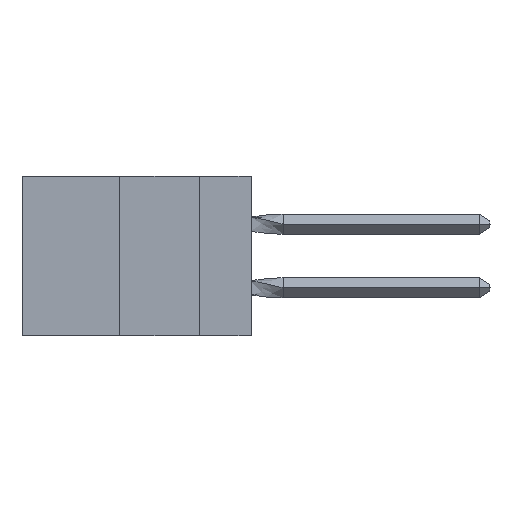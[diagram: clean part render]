
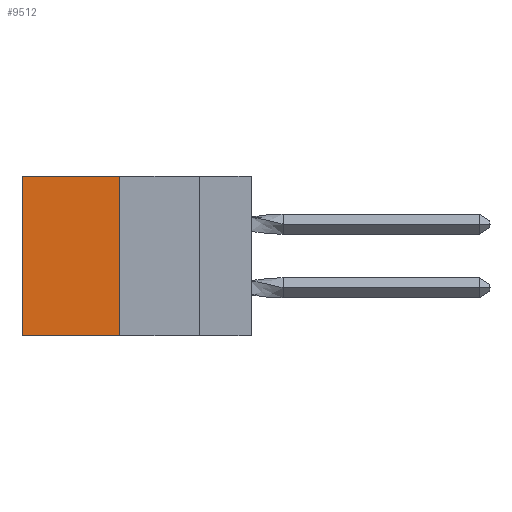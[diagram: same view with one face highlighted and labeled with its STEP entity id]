
A CAD part, left-side view. The second image highlights one B-rep face of the part: STEP entity #9512.
In plain terms, the highlighted planar face has unit normal (-1, 0, 0).
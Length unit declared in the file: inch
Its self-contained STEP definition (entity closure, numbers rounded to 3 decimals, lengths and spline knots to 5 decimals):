
#58 = VERTEX_POINT ( 'NONE', #33733 ) ;
#364 = CARTESIAN_POINT ( 'NONE',  ( 0.305, 0.413, 0. ) ) ;
#614 = PLANE ( 'NONE',  #31232 ) ;
#2203 = EDGE_CURVE ( 'NONE', #58, #4278, #3435, .T. ) ;
#2851 = DIRECTION ( 'NONE',  ( 1., 0., 0. ) ) ;
#3077 = DIRECTION ( 'NONE',  ( 0., 0., -1. ) ) ;
#3435 = LINE ( 'NONE', #13262, #12978 ) ;
#4278 = VERTEX_POINT ( 'NONE', #6064 ) ;
#4628 = CARTESIAN_POINT ( 'NONE',  ( 0.305, 0.72, -0.5 ) ) ;
#5631 = EDGE_CURVE ( 'NONE', #26437, #21655, #18759, .T. ) ;
#6064 = CARTESIAN_POINT ( 'NONE',  ( 0.305, 0.413, -0.5 ) ) ;
#6099 = FACE_OUTER_BOUND ( 'NONE', #22863, .T. ) ;
#6787 = CARTESIAN_POINT ( 'NONE',  ( 0.305, 0.72, 0. ) ) ;
#9512 = ADVANCED_FACE ( 'NONE', ( #6099 ), #614, .F. ) ;
#11023 = CARTESIAN_POINT ( 'NONE',  ( 0.305, 0.413, -0.5 ) ) ;
#11597 = VECTOR ( 'NONE', #33432, 39.37008 ) ;
#12978 = VECTOR ( 'NONE', #21033, 39.37008 ) ;
#13262 = CARTESIAN_POINT ( 'NONE',  ( 0.305, 0.413, -0.5 ) ) ;
#13399 = EDGE_CURVE ( 'NONE', #4278, #21655, #34702, .T. ) ;
#15177 = EDGE_CURVE ( 'NONE', #58, #26437, #20673, .T. ) ;
#17017 = CARTESIAN_POINT ( 'NONE',  ( 0.305, 0.72, -0.5 ) ) ;
#18759 = LINE ( 'NONE', #17017, #11597 ) ;
#19691 = CARTESIAN_POINT ( 'NONE',  ( 0.305, 0.413, -0.5 ) ) ;
#20673 = LINE ( 'NONE', #364, #21968 ) ;
#21033 = DIRECTION ( 'NONE',  ( 0., 0., -1. ) ) ;
#21655 = VERTEX_POINT ( 'NONE', #4628 ) ;
#21968 = VECTOR ( 'NONE', #24506, 39.37008 ) ;
#22863 = EDGE_LOOP ( 'NONE', ( #26776, #24347, #32426, #28877 ) ) ;
#24347 = ORIENTED_EDGE ( 'NONE', *, *, #13399, .F. ) ;
#24506 = DIRECTION ( 'NONE',  ( 0., 1., 0. ) ) ;
#26437 = VERTEX_POINT ( 'NONE', #6787 ) ;
#26776 = ORIENTED_EDGE ( 'NONE', *, *, #5631, .T. ) ;
#28123 = DIRECTION ( 'NONE',  ( 0., 1., 0. ) ) ;
#28773 = VECTOR ( 'NONE', #28123, 39.37008 ) ;
#28877 = ORIENTED_EDGE ( 'NONE', *, *, #15177, .T. ) ;
#31232 = AXIS2_PLACEMENT_3D ( 'NONE', #11023, #2851, #3077 ) ;
#32426 = ORIENTED_EDGE ( 'NONE', *, *, #2203, .F. ) ;
#33432 = DIRECTION ( 'NONE',  ( 0., 0., -1. ) ) ;
#33733 = CARTESIAN_POINT ( 'NONE',  ( 0.305, 0.413, 0. ) ) ;
#34702 = LINE ( 'NONE', #19691, #28773 ) ;
